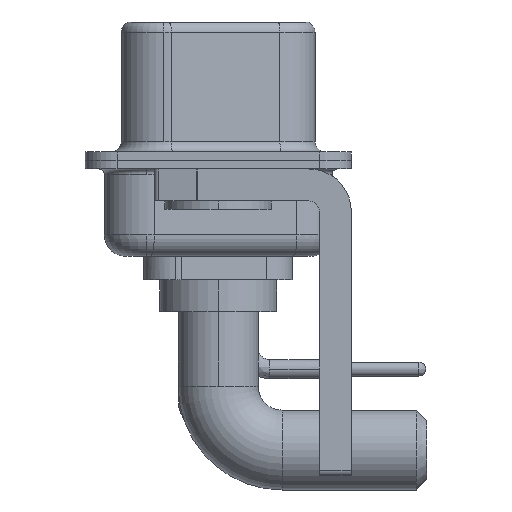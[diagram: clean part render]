
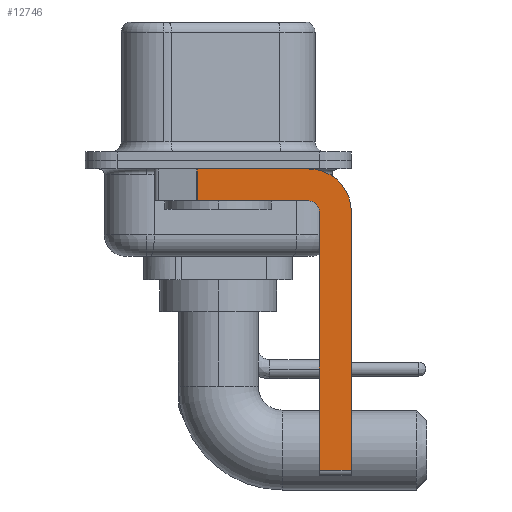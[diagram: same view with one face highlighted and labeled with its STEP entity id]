
A CAD part, left-side view. The second image highlights one B-rep face of the part: STEP entity #12746.
In plain terms, the highlighted planar face has unit normal (-1, 0, 0).
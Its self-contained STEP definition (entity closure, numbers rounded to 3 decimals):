
#32 = CARTESIAN_POINT ( 'NONE',  ( -2.9, -4.25, -1.9 ) ) ;
#532 = VECTOR ( 'NONE', #22669, 1000. ) ;
#552 = ORIENTED_EDGE ( 'NONE', *, *, #10141, .T. ) ;
#789 = EDGE_CURVE ( 'NONE', #2201, #10504, #14170, .T. ) ;
#1580 = VERTEX_POINT ( 'NONE', #32 ) ;
#1668 = CARTESIAN_POINT ( 'NONE',  ( -2.9, -4.25, -2.4 ) ) ;
#1783 = EDGE_CURVE ( 'NONE', #16740, #8448, #8295, .T. ) ;
#1855 = EDGE_CURVE ( 'NONE', #2201, #20698, #5085, .T. ) ;
#2201 = VERTEX_POINT ( 'NONE', #4570 ) ;
#2597 = ORIENTED_EDGE ( 'NONE', *, *, #7351, .F. ) ;
#2811 = CARTESIAN_POINT ( 'NONE',  ( -2.9, -6.25, -2.4 ) ) ;
#3166 = DIRECTION ( 'NONE',  ( 0., -1., 0. ) ) ;
#3320 = VECTOR ( 'NONE', #5199, 1000. ) ;
#3721 = ORIENTED_EDGE ( 'NONE', *, *, #24175, .F. ) ;
#4078 = CARTESIAN_POINT ( 'NONE',  ( -2.9, -4.75, -2.4 ) ) ;
#4570 = CARTESIAN_POINT ( 'NONE',  ( -2.9, -4.75, -14.55 ) ) ;
#5079 = CARTESIAN_POINT ( 'NONE',  ( -2.9, -4.25, -2.4 ) ) ;
#5085 = LINE ( 'NONE', #18515, #3320 ) ;
#5199 = DIRECTION ( 'NONE',  ( 0., 0., 1. ) ) ;
#5503 = DIRECTION ( 'NONE',  ( 1., 0., 0. ) ) ;
#5724 = CIRCLE ( 'NONE', #22636, 2. ) ;
#5738 = ORIENTED_EDGE ( 'NONE', *, *, #1783, .F. ) ;
#6853 = CIRCLE ( 'NONE', #7647, 0.5 ) ;
#7044 = CARTESIAN_POINT ( 'NONE',  ( -2.9, -4.25, -2.4 ) ) ;
#7351 = EDGE_CURVE ( 'NONE', #8448, #21245, #5724, .T. ) ;
#7647 = AXIS2_PLACEMENT_3D ( 'NONE', #5079, #12623, #20109 ) ;
#8295 = LINE ( 'NONE', #14229, #19876 ) ;
#8306 = DIRECTION ( 'NONE',  ( 0., 0., -1. ) ) ;
#8409 = CARTESIAN_POINT ( 'NONE',  ( -2.9, -6.25, -14.55 ) ) ;
#8448 = VERTEX_POINT ( 'NONE', #13269 ) ;
#9293 = LINE ( 'NONE', #16705, #11341 ) ;
#9850 = VECTOR ( 'NONE', #11836, 1000. ) ;
#10141 = EDGE_CURVE ( 'NONE', #16740, #18916, #9293, .T. ) ;
#10504 = VERTEX_POINT ( 'NONE', #8409 ) ;
#10672 = DIRECTION ( 'NONE',  ( 0., 0., -1. ) ) ;
#11341 = VECTOR ( 'NONE', #10672, 1000. ) ;
#11543 = CARTESIAN_POINT ( 'NONE',  ( -2.9, 0.978, -1.9 ) ) ;
#11667 = CARTESIAN_POINT ( 'NONE',  ( -2.9, 0.978, -0.4 ) ) ;
#11836 = DIRECTION ( 'NONE',  ( 0., 1., 0. ) ) ;
#12262 = DIRECTION ( 'NONE',  ( 0., -1., 0. ) ) ;
#12383 = EDGE_CURVE ( 'NONE', #1580, #18916, #17497, .T. ) ;
#12411 = LINE ( 'NONE', #20584, #532 ) ;
#12623 = DIRECTION ( 'NONE',  ( -1., 0., 0. ) ) ;
#12643 = AXIS2_PLACEMENT_3D ( 'NONE', #1668, #5503, #20660 ) ;
#12746 = ADVANCED_FACE ( 'NONE', ( #24220 ), #19055, .F. ) ;
#13269 = CARTESIAN_POINT ( 'NONE',  ( -2.9, -4.25, -0.4 ) ) ;
#13938 = VECTOR ( 'NONE', #3166, 1000. ) ;
#14170 = LINE ( 'NONE', #17865, #13938 ) ;
#14188 = EDGE_LOOP ( 'NONE', ( #5738, #552, #24341, #3721, #14235, #23649, #23170, #2597 ) ) ;
#14229 = CARTESIAN_POINT ( 'NONE',  ( -2.9, 3., -0.4 ) ) ;
#14235 = ORIENTED_EDGE ( 'NONE', *, *, #1855, .F. ) ;
#16705 = CARTESIAN_POINT ( 'NONE',  ( -2.9, 0.978, -1.9 ) ) ;
#16740 = VERTEX_POINT ( 'NONE', #11667 ) ;
#17446 = DIRECTION ( 'NONE',  ( 1., 0., 0. ) ) ;
#17497 = LINE ( 'NONE', #23126, #9850 ) ;
#17865 = CARTESIAN_POINT ( 'NONE',  ( -2.9, -4.25, -14.55 ) ) ;
#17949 = EDGE_CURVE ( 'NONE', #21245, #10504, #12411, .T. ) ;
#18515 = CARTESIAN_POINT ( 'NONE',  ( -2.9, -4.75, -14.8 ) ) ;
#18916 = VERTEX_POINT ( 'NONE', #11543 ) ;
#19055 = PLANE ( 'NONE',  #12643 ) ;
#19876 = VECTOR ( 'NONE', #12262, 1000. ) ;
#20109 = DIRECTION ( 'NONE',  ( 0., 0., 1. ) ) ;
#20584 = CARTESIAN_POINT ( 'NONE',  ( -2.9, -6.25, -2.4 ) ) ;
#20660 = DIRECTION ( 'NONE',  ( 0., 0., -1. ) ) ;
#20698 = VERTEX_POINT ( 'NONE', #4078 ) ;
#21245 = VERTEX_POINT ( 'NONE', #2811 ) ;
#22636 = AXIS2_PLACEMENT_3D ( 'NONE', #7044, #17446, #8306 ) ;
#22669 = DIRECTION ( 'NONE',  ( 0., 0., -1. ) ) ;
#23126 = CARTESIAN_POINT ( 'NONE',  ( -2.9, -4.25, -1.9 ) ) ;
#23170 = ORIENTED_EDGE ( 'NONE', *, *, #17949, .F. ) ;
#23649 = ORIENTED_EDGE ( 'NONE', *, *, #789, .T. ) ;
#24175 = EDGE_CURVE ( 'NONE', #20698, #1580, #6853, .T. ) ;
#24220 = FACE_OUTER_BOUND ( 'NONE', #14188, .T. ) ;
#24341 = ORIENTED_EDGE ( 'NONE', *, *, #12383, .F. ) ;
